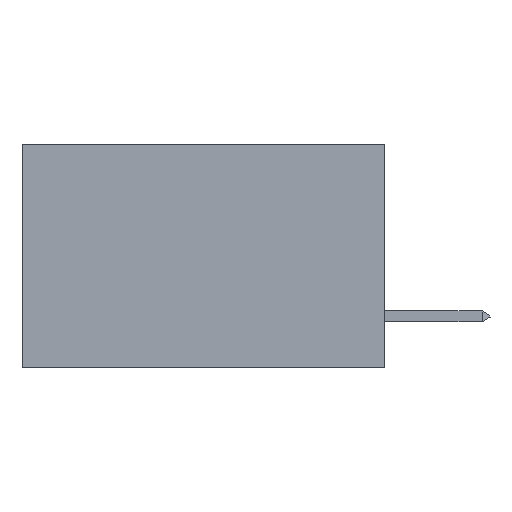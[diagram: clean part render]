
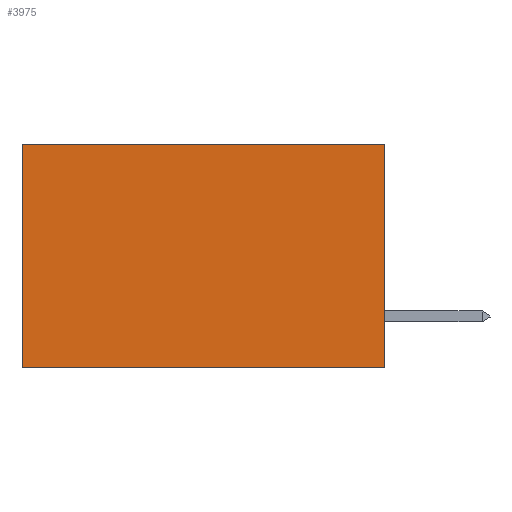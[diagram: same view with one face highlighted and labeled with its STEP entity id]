
A CAD part, left-side view. The second image highlights one B-rep face of the part: STEP entity #3975.
In plain terms, the highlighted planar face has unit normal (-1, 0, 0).
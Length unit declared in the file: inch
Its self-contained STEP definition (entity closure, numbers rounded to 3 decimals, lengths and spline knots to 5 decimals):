
#117 = EDGE_CURVE ( 'NONE', #5794, #10935, #1630, .T. ) ;
#640 = VECTOR ( 'NONE', #6629, 39.37008 ) ;
#651 = PLANE ( 'NONE',  #837 ) ;
#837 = AXIS2_PLACEMENT_3D ( 'NONE', #1738, #1596, #2868 ) ;
#1323 = VERTEX_POINT ( 'NONE', #10488 ) ;
#1596 = DIRECTION ( 'NONE',  ( 1., 0., 0. ) ) ;
#1630 = LINE ( 'NONE', #9557, #12912 ) ;
#1723 = LINE ( 'NONE', #13343, #4152 ) ;
#1738 = CARTESIAN_POINT ( 'NONE',  ( 0.2875, 0., 0. ) ) ;
#2401 = VERTEX_POINT ( 'NONE', #14128 ) ;
#2565 = CARTESIAN_POINT ( 'NONE',  ( 0.2875, 0., -0.37 ) ) ;
#2707 = ORIENTED_EDGE ( 'NONE', *, *, #117, .F. ) ;
#2823 = DIRECTION ( 'NONE',  ( 0., 0., -1. ) ) ;
#2868 = DIRECTION ( 'NONE',  ( 0., 0., -1. ) ) ;
#3408 = EDGE_LOOP ( 'NONE', ( #7990, #6588, #2707, #3898 ) ) ;
#3898 = ORIENTED_EDGE ( 'NONE', *, *, #13829, .T. ) ;
#3975 = ADVANCED_FACE ( 'NONE', ( #9915 ), #651, .F. ) ;
#4095 = LINE ( 'NONE', #14142, #640 ) ;
#4152 = VECTOR ( 'NONE', #2823, 39.37008 ) ;
#4187 = DIRECTION ( 'NONE',  ( 0., 0., -1. ) ) ;
#5794 = VERTEX_POINT ( 'NONE', #13121 ) ;
#5914 = EDGE_CURVE ( 'NONE', #1323, #2401, #1723, .T. ) ;
#6319 = CARTESIAN_POINT ( 'NONE',  ( 0.2875, 0., -0.37 ) ) ;
#6588 = ORIENTED_EDGE ( 'NONE', *, *, #13487, .F. ) ;
#6629 = DIRECTION ( 'NONE',  ( 0., 1., 0. ) ) ;
#7990 = ORIENTED_EDGE ( 'NONE', *, *, #5914, .T. ) ;
#9557 = CARTESIAN_POINT ( 'NONE',  ( 0.2875, 0., 0. ) ) ;
#9915 = FACE_OUTER_BOUND ( 'NONE', #3408, .T. ) ;
#10488 = CARTESIAN_POINT ( 'NONE',  ( 0.2875, 0.6, 0. ) ) ;
#10762 = VECTOR ( 'NONE', #12306, 39.37008 ) ;
#10935 = VERTEX_POINT ( 'NONE', #2565 ) ;
#11261 = LINE ( 'NONE', #6319, #10762 ) ;
#12306 = DIRECTION ( 'NONE',  ( 0., 1., 0. ) ) ;
#12912 = VECTOR ( 'NONE', #4187, 39.37008 ) ;
#13121 = CARTESIAN_POINT ( 'NONE',  ( 0.2875, 0., 0. ) ) ;
#13343 = CARTESIAN_POINT ( 'NONE',  ( 0.2875, 0.6, 0. ) ) ;
#13487 = EDGE_CURVE ( 'NONE', #10935, #2401, #11261, .T. ) ;
#13829 = EDGE_CURVE ( 'NONE', #5794, #1323, #4095, .T. ) ;
#14128 = CARTESIAN_POINT ( 'NONE',  ( 0.2875, 0.6, -0.37 ) ) ;
#14142 = CARTESIAN_POINT ( 'NONE',  ( 0.2875, 0., 0. ) ) ;
